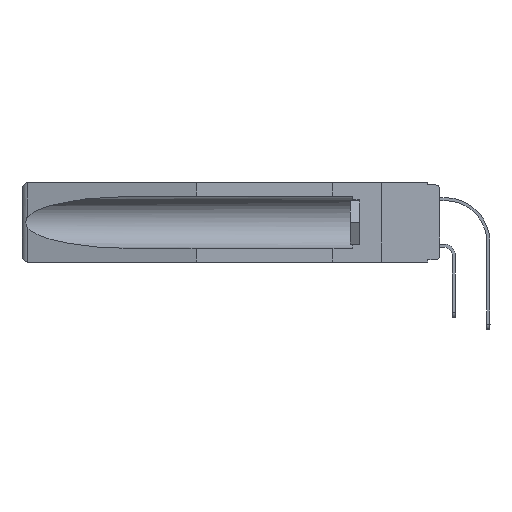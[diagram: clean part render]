
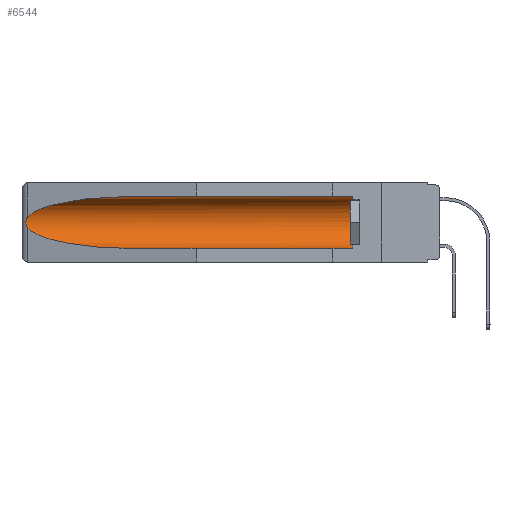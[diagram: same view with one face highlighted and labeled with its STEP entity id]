
A CAD part, left-side view. The second image highlights one B-rep face of the part: STEP entity #6544.
In plain terms, the highlighted cylindrical face has radius 2.857 mm (diameter 5.715 mm), a partial arc.
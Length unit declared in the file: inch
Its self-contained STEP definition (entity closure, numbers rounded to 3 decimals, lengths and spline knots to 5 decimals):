
#83 = CARTESIAN_POINT ( 'NONE',  ( 0.2673, 1.53269, -0.17917 ) ) ;
#140 = CARTESIAN_POINT ( 'NONE',  ( 0.26537, 1.52718, -0.19328 ) ) ;
#929 = VECTOR ( 'NONE', #13785, 39.37008 ) ;
#1239 = VERTEX_POINT ( 'NONE', #16038 ) ;
#1253 = CARTESIAN_POINT ( 'NONE',  ( 0.26654, 1.53092, -0.15636 ) ) ;
#1335 = VERTEX_POINT ( 'NONE', #4646 ) ;
#1462 = DIRECTION ( 'NONE',  ( 0., 1., 0. ) ) ;
#1646 = CARTESIAN_POINT ( 'NONE',  ( 0.155, 1.07973, -0.059 ) ) ;
#1962 = VERTEX_POINT ( 'NONE', #13751 ) ;
#2012 = ORIENTED_EDGE ( 'NONE', *, *, #13959, .T. ) ;
#2025 = LINE ( 'NONE', #7905, #929 ) ;
#2295 = CARTESIAN_POINT ( 'NONE',  ( 0.26537, 1.52718, -0.19328 ) ) ;
#2423 = CARTESIAN_POINT ( 'NONE',  ( 0.155, 0.126, -0.059 ) ) ;
#2593 = EDGE_CURVE ( 'NONE', #4218, #1239, #13418, .T. ) ;
#3831 = CARTESIAN_POINT ( 'NONE',  ( 0.21114, 1.30732, -0.284 ) ) ;
#3929 = CARTESIAN_POINT ( 'NONE',  ( 0.155, 1.07973, -0.284 ) ) ;
#4218 = VERTEX_POINT ( 'NONE', #2423 ) ;
#4514 = CARTESIAN_POINT ( 'NONE',  ( 0.26655, 1.53094, -0.18657 ) ) ;
#4580 = EDGE_CURVE ( 'NONE', #1335, #10379, #2025, .T. ) ;
#4646 = CARTESIAN_POINT ( 'NONE',  ( 0.155, 0.126, -0.284 ) ) ;
#5003 = DIRECTION ( 'NONE',  ( 0., -1., 0. ) ) ;
#5310 = ORIENTED_EDGE ( 'NONE', *, *, #13420, .T. ) ;
#5686 = CARTESIAN_POINT ( 'NONE',  ( 0.26537, 1.52718, -0.14972 ) ) ;
#5873 =( BOUNDED_CURVE ( )  B_SPLINE_CURVE ( 3, ( #2295, #12709, #3831, #3929 ),
 .UNSPECIFIED., .F., .F. ) 
 B_SPLINE_CURVE_WITH_KNOTS ( ( 4, 4 ),
 ( 0.1948, 1.5708 ),
 .UNSPECIFIED. ) 
 CURVE ( )  GEOMETRIC_REPRESENTATION_ITEM ( )  RATIONAL_B_SPLINE_CURVE ( ( 1., 0.848, 0.848, 1. ) ) 
 REPRESENTATION_ITEM ( '' )  );
#5957 = CARTESIAN_POINT ( 'NONE',  ( 0.2673, 1.5327, -0.16383 ) ) ;
#6507 = CARTESIAN_POINT ( 'NONE',  ( 0.155, -0.30754, -0.1715 ) ) ;
#6544 = ADVANCED_FACE ( 'NONE', ( #15122 ), #7974, .F. ) ;
#7218 = CARTESIAN_POINT ( 'NONE',  ( 0.26597, 1.5296, -0.19026 ) ) ;
#7821 = CARTESIAN_POINT ( 'NONE',  ( 0.155, 0.126, -0.1715 ) ) ;
#7858 =( BOUNDED_CURVE ( )  B_SPLINE_CURVE ( 3, ( #1646, #13120, #17641, #5686 ),
 .UNSPECIFIED., .F., .F. ) 
 B_SPLINE_CURVE_WITH_KNOTS ( ( 4, 4 ),
 ( 4.71239, 6.08839 ),
 .UNSPECIFIED. ) 
 CURVE ( )  GEOMETRIC_REPRESENTATION_ITEM ( )  RATIONAL_B_SPLINE_CURVE ( ( 1., 0.848, 0.848, 1. ) ) 
 REPRESENTATION_ITEM ( '' )  );
#7905 = CARTESIAN_POINT ( 'NONE',  ( 0.155, -0.30754, -0.284 ) ) ;
#7974 = CYLINDRICAL_SURFACE ( 'NONE', #11037, 0.1125 ) ;
#8894 = CARTESIAN_POINT ( 'NONE',  ( 0.155, -0.30754, -0.059 ) ) ;
#9332 = AXIS2_PLACEMENT_3D ( 'NONE', #7821, #5003, #16784 ) ;
#10192 = CARTESIAN_POINT ( 'NONE',  ( 0.155, 1.07973, -0.284 ) ) ;
#10313 = CARTESIAN_POINT ( 'NONE',  ( 0.26537, 1.52718, -0.19328 ) ) ;
#10379 = VERTEX_POINT ( 'NONE', #10192 ) ;
#11037 = AXIS2_PLACEMENT_3D ( 'NONE', #6507, #13659, #18196 ) ;
#11760 = EDGE_CURVE ( 'NONE', #1962, #18449, #14410, .T. ) ;
#11856 = CARTESIAN_POINT ( 'NONE',  ( 0.2675, 1.53308, -0.17534 ) ) ;
#12709 = CARTESIAN_POINT ( 'NONE',  ( 0.25451, 1.48313, -0.24835 ) ) ;
#12811 = ORIENTED_EDGE ( 'NONE', *, *, #2593, .T. ) ;
#13120 = CARTESIAN_POINT ( 'NONE',  ( 0.21114, 1.30732, -0.059 ) ) ;
#13418 = LINE ( 'NONE', #8894, #15654 ) ;
#13420 = EDGE_CURVE ( 'NONE', #18449, #10379, #5873, .T. ) ;
#13659 = DIRECTION ( 'NONE',  ( 0., 1., 0. ) ) ;
#13751 = CARTESIAN_POINT ( 'NONE',  ( 0.26537, 1.52718, -0.14972 ) ) ;
#13785 = DIRECTION ( 'NONE',  ( 0., 1., 0. ) ) ;
#13959 = EDGE_CURVE ( 'NONE', #1239, #1962, #7858, .T. ) ;
#14410 = B_SPLINE_CURVE_WITH_KNOTS ( 'NONE', 3,
 ( #14758, #14555, #1253, #5957, #17629, #11856, #83, #4514, #7218, #10313 ),
 .UNSPECIFIED., .F., .F.,
 ( 4, 2, 2, 2, 4 ),
 ( 0., 0.00029, 0.00058, 0.00087, 0.00117 ),
 .UNSPECIFIED. ) ;
#14555 = CARTESIAN_POINT ( 'NONE',  ( 0.26597, 1.52961, -0.15275 ) ) ;
#14758 = CARTESIAN_POINT ( 'NONE',  ( 0.26537, 1.52718, -0.14972 ) ) ;
#15122 = FACE_OUTER_BOUND ( 'NONE', #17521, .T. ) ;
#15445 = EDGE_CURVE ( 'NONE', #1335, #4218, #18515, .T. ) ;
#15654 = VECTOR ( 'NONE', #1462, 39.37008 ) ;
#16038 = CARTESIAN_POINT ( 'NONE',  ( 0.155, 1.07973, -0.059 ) ) ;
#16784 = DIRECTION ( 'NONE',  ( 0., 0., 1. ) ) ;
#17448 = ORIENTED_EDGE ( 'NONE', *, *, #11760, .T. ) ;
#17521 = EDGE_LOOP ( 'NONE', ( #2012, #17448, #5310, #18743, #18524, #12811 ) ) ;
#17629 = CARTESIAN_POINT ( 'NONE',  ( 0.2675, 1.53308, -0.16763 ) ) ;
#17641 = CARTESIAN_POINT ( 'NONE',  ( 0.25451, 1.48313, -0.09465 ) ) ;
#18196 = DIRECTION ( 'NONE',  ( 0., 0., 1. ) ) ;
#18449 = VERTEX_POINT ( 'NONE', #140 ) ;
#18515 = CIRCLE ( 'NONE', #9332, 0.1125 ) ;
#18524 = ORIENTED_EDGE ( 'NONE', *, *, #15445, .T. ) ;
#18743 = ORIENTED_EDGE ( 'NONE', *, *, #4580, .F. ) ;
